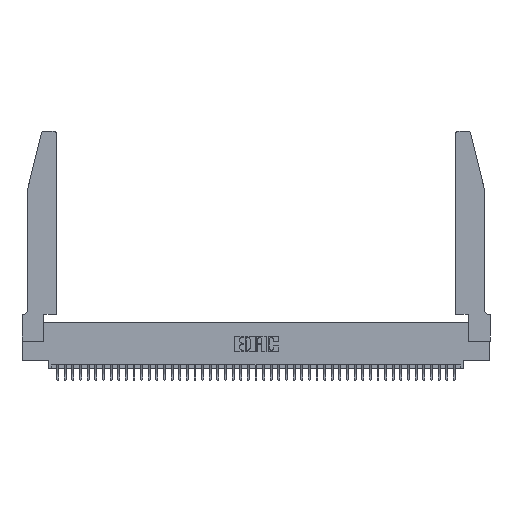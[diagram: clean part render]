
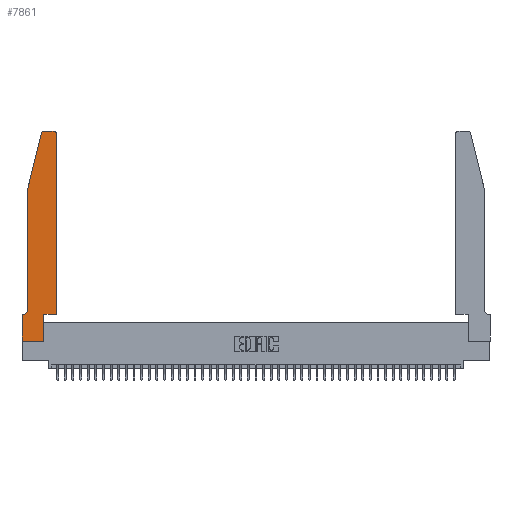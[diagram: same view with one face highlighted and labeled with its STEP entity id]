
A CAD part, top view. The second image highlights one B-rep face of the part: STEP entity #7861.
In plain terms, the highlighted planar face has unit normal (0, 0, 1).
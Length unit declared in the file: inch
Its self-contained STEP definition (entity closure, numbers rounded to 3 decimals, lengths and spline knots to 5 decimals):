
#263 = CARTESIAN_POINT ( 'NONE',  ( 0.4505, 2.72, 0.37 ) ) ;
#286 = VERTEX_POINT ( 'NONE', #13975 ) ;
#1546 = ORIENTED_EDGE ( 'NONE', *, *, #28310, .T. ) ;
#1759 = ORIENTED_EDGE ( 'NONE', *, *, #32216, .T. ) ;
#1969 = CARTESIAN_POINT ( 'NONE',  ( 0.25487, 2.72718, 0.37 ) ) ;
#2071 = CARTESIAN_POINT ( 'NONE',  ( 0., 0., 0.37 ) ) ;
#2944 = VERTEX_POINT ( 'NONE', #7157 ) ;
#3965 = LINE ( 'NONE', #5990, #22653 ) ;
#4148 = FACE_OUTER_BOUND ( 'NONE', #27973, .T. ) ;
#4163 = AXIS2_PLACEMENT_3D ( 'NONE', #11471, #35799, #14966 ) ;
#4860 = ORIENTED_EDGE ( 'NONE', *, *, #24092, .T. ) ;
#5479 = DIRECTION ( 'NONE',  ( 0., -1., 0. ) ) ;
#5587 = DIRECTION ( 'NONE',  ( 0., 0., 1. ) ) ;
#5990 = CARTESIAN_POINT ( 'NONE',  ( 0.4505, 0.35, 0.37 ) ) ;
#5996 = CARTESIAN_POINT ( 'NONE',  ( 0., 0., 0.37 ) ) ;
#6104 = CIRCLE ( 'NONE', #23864, 0.03 ) ;
#6670 = PLANE ( 'NONE',  #20599 ) ;
#6905 = CARTESIAN_POINT ( 'NONE',  ( 0., 0.35, 0.37 ) ) ;
#6972 = EDGE_CURVE ( 'NONE', #12303, #21193, #20721, .T. ) ;
#7157 = CARTESIAN_POINT ( 'NONE',  ( 0.0055, 0.35, 0.37 ) ) ;
#7861 = ADVANCED_FACE ( 'NONE', ( #4148 ), #6670, .T. ) ;
#8439 = LINE ( 'NONE', #28546, #18832 ) ;
#9246 = CARTESIAN_POINT ( 'NONE',  ( 0.2605, 2.75, 0.37 ) ) ;
#9691 = ORIENTED_EDGE ( 'NONE', *, *, #38457, .T. ) ;
#10126 = ORIENTED_EDGE ( 'NONE', *, *, #14335, .T. ) ;
#10165 = CARTESIAN_POINT ( 'NONE',  ( 0.0755, 2., 0.37 ) ) ;
#10234 = DIRECTION ( 'NONE',  ( 0., 0., 1. ) ) ;
#11083 = DIRECTION ( 'NONE',  ( 0., 0., 1. ) ) ;
#11191 = ORIENTED_EDGE ( 'NONE', *, *, #6972, .T. ) ;
#11471 = CARTESIAN_POINT ( 'NONE',  ( 0.0055, 0.42, 0.37 ) ) ;
#12303 = VERTEX_POINT ( 'NONE', #44473 ) ;
#13514 = VERTEX_POINT ( 'NONE', #1969 ) ;
#13532 = VECTOR ( 'NONE', #13680, 39.37008 ) ;
#13680 = DIRECTION ( 'NONE',  ( 0., -1., 0. ) ) ;
#13785 = EDGE_CURVE ( 'NONE', #13514, #44868, #42702, .T. ) ;
#13934 = VECTOR ( 'NONE', #18115, 39.37008 ) ;
#13975 = CARTESIAN_POINT ( 'NONE',  ( 0.4505, 0.35, 0.37 ) ) ;
#13979 = VECTOR ( 'NONE', #34385, 39.37008 ) ;
#14021 = EDGE_CURVE ( 'NONE', #15712, #28393, #32944, .T. ) ;
#14053 = EDGE_CURVE ( 'NONE', #286, #30794, #3965, .T. ) ;
#14335 = EDGE_CURVE ( 'NONE', #2944, #43005, #8439, .T. ) ;
#14720 = VECTOR ( 'NONE', #39489, 39.37008 ) ;
#14966 = DIRECTION ( 'NONE',  ( -1., 0., 0. ) ) ;
#15712 = VERTEX_POINT ( 'NONE', #42743 ) ;
#16358 = ORIENTED_EDGE ( 'NONE', *, *, #25112, .T. ) ;
#17461 = CARTESIAN_POINT ( 'NONE',  ( 0.284, 2.75, 0.37 ) ) ;
#18115 = DIRECTION ( 'NONE',  ( -0.239, -0.971, 0. ) ) ;
#18832 = VECTOR ( 'NONE', #42317, 39.37008 ) ;
#19704 = ORIENTED_EDGE ( 'NONE', *, *, #29851, .T. ) ;
#20599 = AXIS2_PLACEMENT_3D ( 'NONE', #31069, #10234, #34577 ) ;
#20721 = LINE ( 'NONE', #22215, #14720 ) ;
#21193 = VERTEX_POINT ( 'NONE', #30546 ) ;
#21514 = CARTESIAN_POINT ( 'NONE',  ( 0.0755, 2., 0.37 ) ) ;
#22215 = CARTESIAN_POINT ( 'NONE',  ( 0.2865, 0.35, 0.37 ) ) ;
#22653 = VECTOR ( 'NONE', #44202, 39.37008 ) ;
#22819 = LINE ( 'NONE', #10165, #13532 ) ;
#23164 = AXIS2_PLACEMENT_3D ( 'NONE', #31904, #11083, #35417 ) ;
#23705 = VECTOR ( 'NONE', #33593, 39.37008 ) ;
#23708 = EDGE_CURVE ( 'NONE', #25932, #2944, #29265, .T. ) ;
#23864 = AXIS2_PLACEMENT_3D ( 'NONE', #26497, #5587, #30011 ) ;
#24092 = EDGE_CURVE ( 'NONE', #21193, #286, #32472, .T. ) ;
#25112 = EDGE_CURVE ( 'NONE', #43005, #36870, #26930, .T. ) ;
#25932 = VERTEX_POINT ( 'NONE', #34234 ) ;
#26497 = CARTESIAN_POINT ( 'NONE',  ( 0.284, 2.72, 0.37 ) ) ;
#26930 = LINE ( 'NONE', #43694, #44307 ) ;
#27110 = ORIENTED_EDGE ( 'NONE', *, *, #14053, .T. ) ;
#27973 = EDGE_LOOP ( 'NONE', ( #35129, #9691, #38575, #1546, #35085, #10126, #16358, #19704, #11191, #4860, #27110, #1759 ) ) ;
#28310 = EDGE_CURVE ( 'NONE', #44868, #25932, #22819, .T. ) ;
#28393 = VERTEX_POINT ( 'NONE', #17461 ) ;
#28546 = CARTESIAN_POINT ( 'NONE',  ( 0.0755, 0.35, 0.37 ) ) ;
#29265 = CIRCLE ( 'NONE', #4163, 0.07 ) ;
#29851 = EDGE_CURVE ( 'NONE', #36870, #12303, #42698, .T. ) ;
#30011 = DIRECTION ( 'NONE',  ( 1., 0., 0. ) ) ;
#30546 = CARTESIAN_POINT ( 'NONE',  ( 0.2865, 0.35, 0.37 ) ) ;
#30794 = VERTEX_POINT ( 'NONE', #263 ) ;
#31069 = CARTESIAN_POINT ( 'NONE',  ( 0., 0.35, 0.37 ) ) ;
#31904 = CARTESIAN_POINT ( 'NONE',  ( 0.4205, 2.72, 0.37 ) ) ;
#32216 = EDGE_CURVE ( 'NONE', #30794, #15712, #37127, .T. ) ;
#32472 = LINE ( 'NONE', #44668, #13979 ) ;
#32944 = LINE ( 'NONE', #9246, #23705 ) ;
#33509 = VECTOR ( 'NONE', #37377, 39.37008 ) ;
#33593 = DIRECTION ( 'NONE',  ( -1., 0., 0. ) ) ;
#34234 = CARTESIAN_POINT ( 'NONE',  ( 0.0755, 0.42, 0.37 ) ) ;
#34385 = DIRECTION ( 'NONE',  ( 1., 0., 0. ) ) ;
#34577 = DIRECTION ( 'NONE',  ( 1., 0., 0. ) ) ;
#35085 = ORIENTED_EDGE ( 'NONE', *, *, #23708, .T. ) ;
#35129 = ORIENTED_EDGE ( 'NONE', *, *, #14021, .T. ) ;
#35417 = DIRECTION ( 'NONE',  ( 1., 0., 0. ) ) ;
#35799 = DIRECTION ( 'NONE',  ( 0., 0., -1. ) ) ;
#36870 = VERTEX_POINT ( 'NONE', #2071 ) ;
#37127 = CIRCLE ( 'NONE', #23164, 0.03 ) ;
#37377 = DIRECTION ( 'NONE',  ( 1., 0., 0. ) ) ;
#38457 = EDGE_CURVE ( 'NONE', #28393, #13514, #6104, .T. ) ;
#38575 = ORIENTED_EDGE ( 'NONE', *, *, #13785, .T. ) ;
#38921 = CARTESIAN_POINT ( 'NONE',  ( 0.0755, 2., 0.37 ) ) ;
#39489 = DIRECTION ( 'NONE',  ( 0., 1., 0. ) ) ;
#42317 = DIRECTION ( 'NONE',  ( -1., 0., 0. ) ) ;
#42698 = LINE ( 'NONE', #5996, #33509 ) ;
#42702 = LINE ( 'NONE', #38921, #13934 ) ;
#42743 = CARTESIAN_POINT ( 'NONE',  ( 0.4205, 2.75, 0.37 ) ) ;
#43005 = VERTEX_POINT ( 'NONE', #6905 ) ;
#43694 = CARTESIAN_POINT ( 'NONE',  ( 0., 0., 0.37 ) ) ;
#44202 = DIRECTION ( 'NONE',  ( 0., 1., 0. ) ) ;
#44307 = VECTOR ( 'NONE', #5479, 39.37008 ) ;
#44473 = CARTESIAN_POINT ( 'NONE',  ( 0.2865, 0., 0.37 ) ) ;
#44668 = CARTESIAN_POINT ( 'NONE',  ( 0.4505, 0.35, 0.37 ) ) ;
#44868 = VERTEX_POINT ( 'NONE', #21514 ) ;
